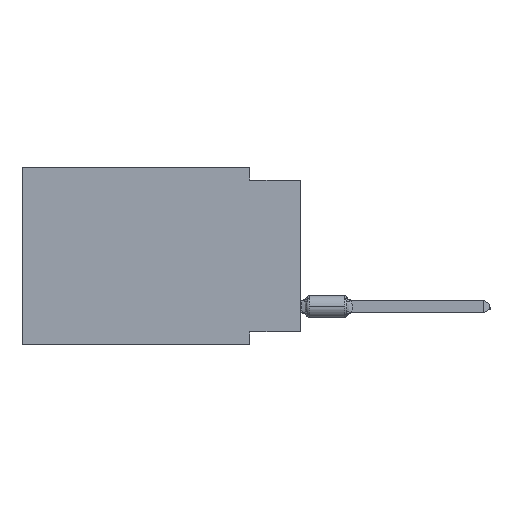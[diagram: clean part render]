
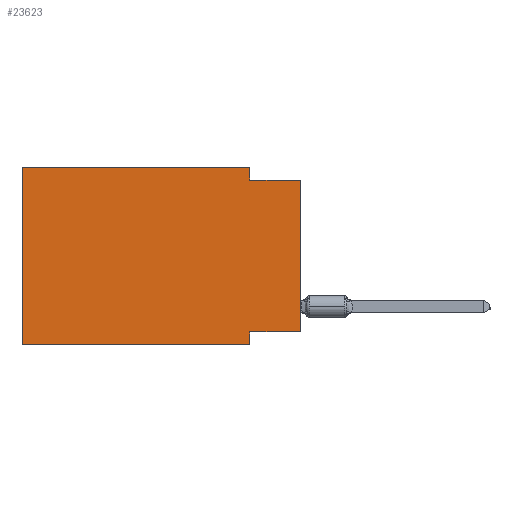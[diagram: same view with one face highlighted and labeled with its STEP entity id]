
A CAD part, left-side view. The second image highlights one B-rep face of the part: STEP entity #23623.
In plain terms, the highlighted planar face has unit normal (-1, 0, 0).
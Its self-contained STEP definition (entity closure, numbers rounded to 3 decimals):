
#504 = CARTESIAN_POINT ( 'NONE',  ( 0., 0., 0. ) ) ;
#949 = VERTEX_POINT ( 'NONE', #4412 ) ;
#1648 = ORIENTED_EDGE ( 'NONE', *, *, #31468, .T. ) ;
#2339 = LINE ( 'NONE', #15660, #16977 ) ;
#2713 = EDGE_CURVE ( 'NONE', #25503, #33807, #25686, .T. ) ;
#3509 = LINE ( 'NONE', #14348, #6414 ) ;
#4208 = CARTESIAN_POINT ( 'NONE',  ( 0., 0., -0.635 ) ) ;
#4412 = CARTESIAN_POINT ( 'NONE',  ( 0., 13.97, -8.89 ) ) ;
#4848 = AXIS2_PLACEMENT_3D ( 'NONE', #13634, #10606, #21417 ) ;
#5651 = ORIENTED_EDGE ( 'NONE', *, *, #16897, .F. ) ;
#5715 = ORIENTED_EDGE ( 'NONE', *, *, #31618, .F. ) ;
#6020 = EDGE_CURVE ( 'NONE', #949, #25503, #21027, .T. ) ;
#6055 = VECTOR ( 'NONE', #30977, 1000. ) ;
#6414 = VECTOR ( 'NONE', #11672, 1000. ) ;
#7222 = DIRECTION ( 'NONE',  ( 0., -1., 0. ) ) ;
#8032 = DIRECTION ( 'NONE',  ( 0., 1., 0. ) ) ;
#8483 = FACE_OUTER_BOUND ( 'NONE', #15180, .T. ) ;
#8868 = VERTEX_POINT ( 'NONE', #25712 ) ;
#10059 = CARTESIAN_POINT ( 'NONE',  ( 0., 13.97, 0. ) ) ;
#10606 = DIRECTION ( 'NONE',  ( 1., 0., 0. ) ) ;
#10981 = LINE ( 'NONE', #504, #29049 ) ;
#11255 = ORIENTED_EDGE ( 'NONE', *, *, #6020, .F. ) ;
#11672 = DIRECTION ( 'NONE',  ( 0., -1., 0. ) ) ;
#12343 = CARTESIAN_POINT ( 'NONE',  ( 0., 13.97, 0. ) ) ;
#12352 = CARTESIAN_POINT ( 'NONE',  ( 0., 13.97, -8.89 ) ) ;
#12782 = EDGE_CURVE ( 'NONE', #27506, #19298, #2339, .T. ) ;
#13634 = CARTESIAN_POINT ( 'NONE',  ( 0., 13.97, 0. ) ) ;
#13795 = CARTESIAN_POINT ( 'NONE',  ( 0., 0., -8.255 ) ) ;
#13821 = PLANE ( 'NONE',  #4848 ) ;
#14348 = CARTESIAN_POINT ( 'NONE',  ( 0., 0., -0.635 ) ) ;
#14844 = LINE ( 'NONE', #31159, #6055 ) ;
#14995 = DIRECTION ( 'NONE',  ( 0., 0., -1. ) ) ;
#15139 = CARTESIAN_POINT ( 'NONE',  ( 0., 13.97, 0. ) ) ;
#15180 = EDGE_LOOP ( 'NONE', ( #1648, #5715, #19914, #17452, #11255, #16874, #5651, #19902 ) ) ;
#15660 = CARTESIAN_POINT ( 'NONE',  ( 0., 0., -8.255 ) ) ;
#16874 = ORIENTED_EDGE ( 'NONE', *, *, #34221, .T. ) ;
#16897 = EDGE_CURVE ( 'NONE', #19298, #8868, #14844, .T. ) ;
#16977 = VECTOR ( 'NONE', #8032, 1000. ) ;
#17149 = CARTESIAN_POINT ( 'NONE',  ( 0., 2.54, 0. ) ) ;
#17316 = LINE ( 'NONE', #17149, #29078 ) ;
#17452 = ORIENTED_EDGE ( 'NONE', *, *, #2713, .F. ) ;
#18204 = LINE ( 'NONE', #12352, #35074 ) ;
#19298 = VERTEX_POINT ( 'NONE', #24515 ) ;
#19494 = DIRECTION ( 'NONE',  ( 0., 0., 1. ) ) ;
#19902 = ORIENTED_EDGE ( 'NONE', *, *, #12782, .F. ) ;
#19914 = ORIENTED_EDGE ( 'NONE', *, *, #30007, .F. ) ;
#21027 = LINE ( 'NONE', #12343, #31648 ) ;
#21417 = DIRECTION ( 'NONE',  ( 0., 0., -1. ) ) ;
#23277 = CARTESIAN_POINT ( 'NONE',  ( 0., 2.54, 0. ) ) ;
#23623 = ADVANCED_FACE ( 'NONE', ( #8483 ), #13821, .F. ) ;
#24515 = CARTESIAN_POINT ( 'NONE',  ( 0., 2.54, -8.255 ) ) ;
#25503 = VERTEX_POINT ( 'NONE', #15139 ) ;
#25686 = LINE ( 'NONE', #10059, #27469 ) ;
#25712 = CARTESIAN_POINT ( 'NONE',  ( 0., 2.54, -8.89 ) ) ;
#27469 = VECTOR ( 'NONE', #7222, 1000. ) ;
#27506 = VERTEX_POINT ( 'NONE', #13795 ) ;
#28416 = VERTEX_POINT ( 'NONE', #4208 ) ;
#29018 = CARTESIAN_POINT ( 'NONE',  ( 0., 2.54, -0.635 ) ) ;
#29049 = VECTOR ( 'NONE', #19494, 1000. ) ;
#29078 = VECTOR ( 'NONE', #14995, 1000. ) ;
#30007 = EDGE_CURVE ( 'NONE', #33807, #34279, #17316, .T. ) ;
#30977 = DIRECTION ( 'NONE',  ( 0., 0., -1. ) ) ;
#31159 = CARTESIAN_POINT ( 'NONE',  ( 0., 2.54, -8.89 ) ) ;
#31161 = DIRECTION ( 'NONE',  ( 0., -1., 0. ) ) ;
#31468 = EDGE_CURVE ( 'NONE', #27506, #28416, #10981, .T. ) ;
#31618 = EDGE_CURVE ( 'NONE', #34279, #28416, #3509, .T. ) ;
#31648 = VECTOR ( 'NONE', #31848, 1000. ) ;
#31848 = DIRECTION ( 'NONE',  ( 0., 0., 1. ) ) ;
#33807 = VERTEX_POINT ( 'NONE', #23277 ) ;
#34221 = EDGE_CURVE ( 'NONE', #949, #8868, #18204, .T. ) ;
#34279 = VERTEX_POINT ( 'NONE', #29018 ) ;
#35074 = VECTOR ( 'NONE', #31161, 1000. ) ;
